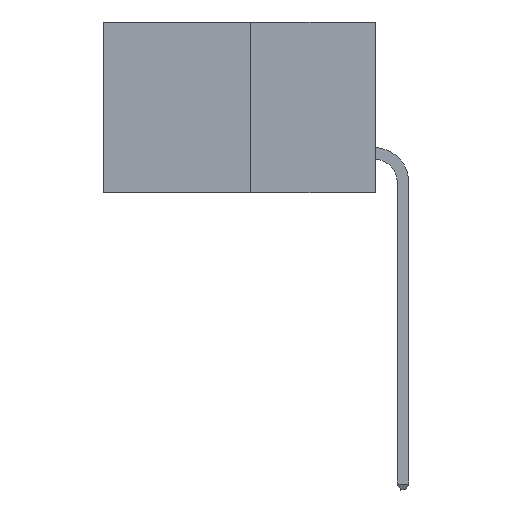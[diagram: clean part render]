
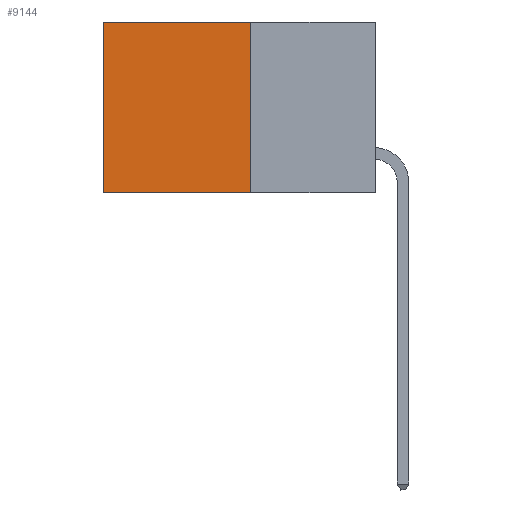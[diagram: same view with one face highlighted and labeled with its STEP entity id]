
A CAD part, left-side view. The second image highlights one B-rep face of the part: STEP entity #9144.
In plain terms, the highlighted planar face has unit normal (-1, 0, 0).
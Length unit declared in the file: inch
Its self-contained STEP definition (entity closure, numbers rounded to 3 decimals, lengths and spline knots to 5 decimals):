
#140 = DIRECTION ( 'NONE',  ( 0., 0., -1. ) ) ;
#275 = CARTESIAN_POINT ( 'NONE',  ( 0.277, 0.27, -0.37 ) ) ;
#1282 = DIRECTION ( 'NONE',  ( 0., 0., -1. ) ) ;
#1725 = LINE ( 'NONE', #4046, #8762 ) ;
#2070 = VERTEX_POINT ( 'NONE', #17913 ) ;
#2108 = CARTESIAN_POINT ( 'NONE',  ( 0.277, 0.27, 0. ) ) ;
#2607 = DIRECTION ( 'NONE',  ( 0., 1., 0. ) ) ;
#2715 = CARTESIAN_POINT ( 'NONE',  ( 0.277, 0.59, -0.37 ) ) ;
#4046 = CARTESIAN_POINT ( 'NONE',  ( 0.277, 0.27, -0.37 ) ) ;
#4383 = VECTOR ( 'NONE', #13346, 39.37008 ) ;
#4677 = CARTESIAN_POINT ( 'NONE',  ( 0.277, 0.59, -0.37 ) ) ;
#5141 = CARTESIAN_POINT ( 'NONE',  ( 0.277, 0.59, 0. ) ) ;
#6042 = EDGE_LOOP ( 'NONE', ( #16544, #13319, #8226, #11610 ) ) ;
#6668 = EDGE_CURVE ( 'NONE', #2070, #17825, #7143, .T. ) ;
#7143 = LINE ( 'NONE', #275, #17793 ) ;
#7795 = LINE ( 'NONE', #2715, #13857 ) ;
#8070 = LINE ( 'NONE', #2108, #4383 ) ;
#8226 = ORIENTED_EDGE ( 'NONE', *, *, #6668, .F. ) ;
#8287 = VERTEX_POINT ( 'NONE', #5141 ) ;
#8762 = VECTOR ( 'NONE', #2607, 39.37008 ) ;
#9144 = ADVANCED_FACE ( 'NONE', ( #13375 ), #15826, .F. ) ;
#11610 = ORIENTED_EDGE ( 'NONE', *, *, #12184, .T. ) ;
#12027 = VERTEX_POINT ( 'NONE', #4677 ) ;
#12184 = EDGE_CURVE ( 'NONE', #2070, #8287, #8070, .T. ) ;
#13319 = ORIENTED_EDGE ( 'NONE', *, *, #14618, .F. ) ;
#13346 = DIRECTION ( 'NONE',  ( 0., 1., 0. ) ) ;
#13375 = FACE_OUTER_BOUND ( 'NONE', #6042, .T. ) ;
#13857 = VECTOR ( 'NONE', #1282, 39.37008 ) ;
#14618 = EDGE_CURVE ( 'NONE', #17825, #12027, #1725, .T. ) ;
#15564 = CARTESIAN_POINT ( 'NONE',  ( 0.277, 0.27, -0.37 ) ) ;
#15707 = DIRECTION ( 'NONE',  ( 0., 0., -1. ) ) ;
#15748 = DIRECTION ( 'NONE',  ( 1., 0., 0. ) ) ;
#15806 = CARTESIAN_POINT ( 'NONE',  ( 0.277, 0.27, -0.37 ) ) ;
#15826 = PLANE ( 'NONE',  #17087 ) ;
#16437 = EDGE_CURVE ( 'NONE', #8287, #12027, #7795, .T. ) ;
#16544 = ORIENTED_EDGE ( 'NONE', *, *, #16437, .T. ) ;
#17087 = AXIS2_PLACEMENT_3D ( 'NONE', #15806, #15748, #15707 ) ;
#17793 = VECTOR ( 'NONE', #140, 39.37008 ) ;
#17825 = VERTEX_POINT ( 'NONE', #15564 ) ;
#17913 = CARTESIAN_POINT ( 'NONE',  ( 0.277, 0.27, 0. ) ) ;
